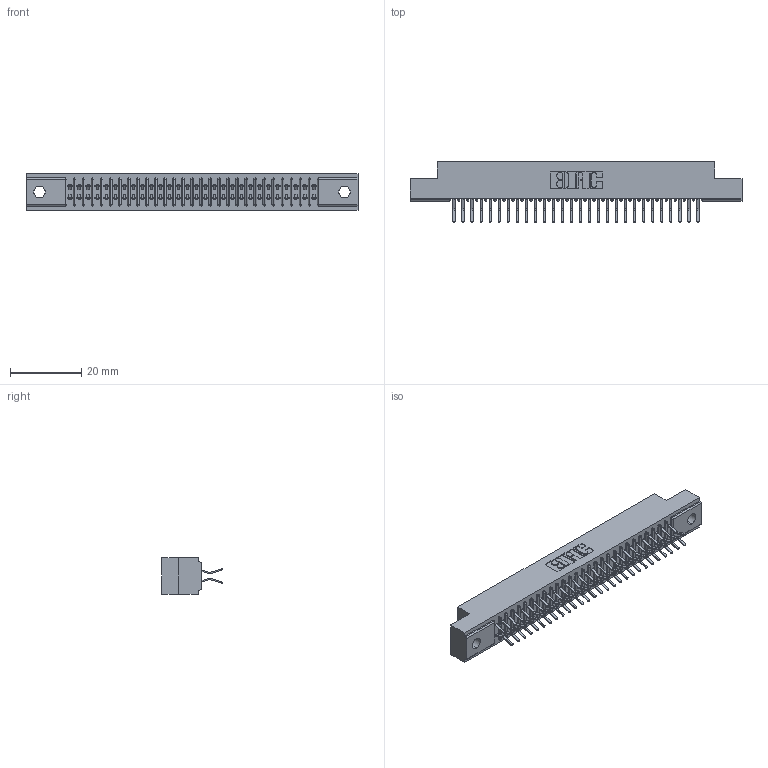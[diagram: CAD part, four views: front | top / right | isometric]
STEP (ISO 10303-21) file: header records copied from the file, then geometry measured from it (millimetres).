
FILE_DESCRIPTION (( 'STEP AP203' ), '1' );
FILE_NAME ('391-056-556-202.STEP', '2018-08-09T11:19:21', ( '' ), ( '' ), 'SwSTEP 2.0', 'SolidWorks 2016', '' );
FILE_SCHEMA (( 'CONFIG_CONTROL_DESIGN' ));
Length unit declared in the file: inch
Products named in the file (3): 341-292-001_341-292-156; 391-056-556-202; 341 Part_.128 (3.25) Dia Mounting Holes
Assembly tree (57 placements, depth 2):
  391-056-556-202
    341 Part_.128 (3.25) Dia Mounting Holes
    341-292-001_341-292-156  x56
Bounding box: 93.34 x 17.07 x 10.16 mm (x, y, z)
Volume: 6858.4 mm3; surface area: 11615.6 mm2
Topology: 57 solids, 57 shells, 4036 faces, 11712 edges, 7598 vertices
Faces by surface type: plane 2308, cylinder 1616, sphere 58, torus 54
Entity records: 35893 total; most frequent: CARTESIAN_POINT 5968, ORIENTED_EDGE 5928, DIRECTION 5806, EDGE_CURVE 2964, LINE 2374, VECTOR 2374, VERTEX_POINT 1878, AXIS2_PLACEMENT_3D 1716
